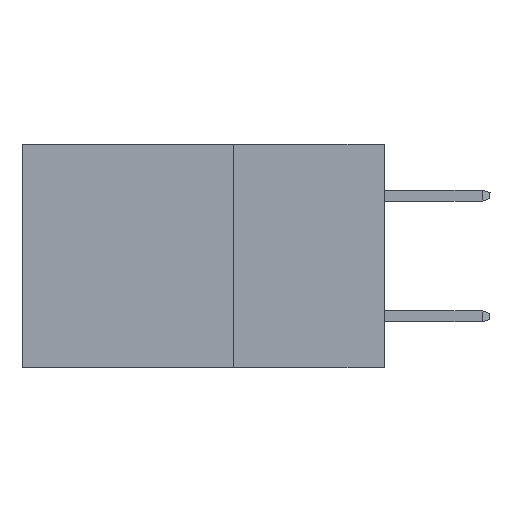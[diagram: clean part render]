
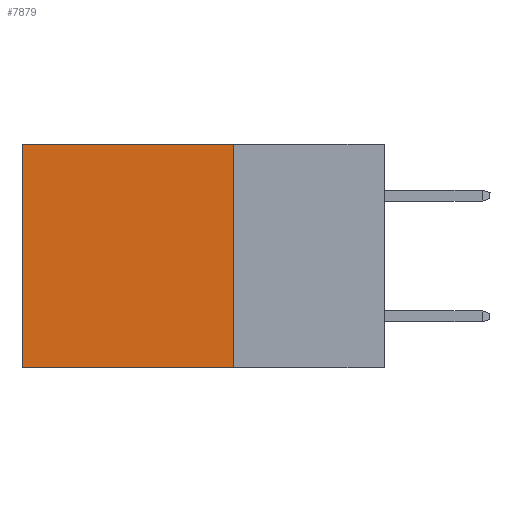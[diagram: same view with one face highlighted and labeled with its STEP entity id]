
A CAD part, left-side view. The second image highlights one B-rep face of the part: STEP entity #7879.
In plain terms, the highlighted planar face has unit normal (-1, 0, 0).
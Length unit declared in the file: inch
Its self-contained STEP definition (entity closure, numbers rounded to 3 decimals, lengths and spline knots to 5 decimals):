
#285 = VECTOR ( 'NONE', #1571, 39.37008 ) ;
#515 = VERTEX_POINT ( 'NONE', #2624 ) ;
#549 = CARTESIAN_POINT ( 'NONE',  ( 0.298, 0.6, -0.37 ) ) ;
#771 = FACE_OUTER_BOUND ( 'NONE', #9081, .T. ) ;
#797 = ORIENTED_EDGE ( 'NONE', *, *, #4668, .T. ) ;
#1075 = CARTESIAN_POINT ( 'NONE',  ( 0.298, 0.25, -0.37 ) ) ;
#1334 = CARTESIAN_POINT ( 'NONE',  ( 0.298, 0.25, 0. ) ) ;
#1498 = CARTESIAN_POINT ( 'NONE',  ( 0.298, 0.25, 0. ) ) ;
#1571 = DIRECTION ( 'NONE',  ( 0., 0., -1. ) ) ;
#1808 = EDGE_CURVE ( 'NONE', #4935, #515, #9360, .T. ) ;
#1875 = PLANE ( 'NONE',  #2362 ) ;
#2045 = DIRECTION ( 'NONE',  ( 0., 1., 0. ) ) ;
#2288 = LINE ( 'NONE', #7924, #6374 ) ;
#2362 = AXIS2_PLACEMENT_3D ( 'NONE', #1334, #10257, #8568 ) ;
#2490 = CARTESIAN_POINT ( 'NONE',  ( 0.298, 0.6, 0. ) ) ;
#2624 = CARTESIAN_POINT ( 'NONE',  ( 0.298, 0.25, -0.37 ) ) ;
#3165 = DIRECTION ( 'NONE',  ( 0., 1., 0. ) ) ;
#4533 = VECTOR ( 'NONE', #2045, 39.37008 ) ;
#4668 = EDGE_CURVE ( 'NONE', #4935, #5518, #2288, .T. ) ;
#4935 = VERTEX_POINT ( 'NONE', #9321 ) ;
#5134 = VERTEX_POINT ( 'NONE', #549 ) ;
#5518 = VERTEX_POINT ( 'NONE', #9917 ) ;
#5830 = ORIENTED_EDGE ( 'NONE', *, *, #1808, .F. ) ;
#6374 = VECTOR ( 'NONE', #3165, 39.37008 ) ;
#7879 = ADVANCED_FACE ( 'NONE', ( #771 ), #1875, .F. ) ;
#7924 = CARTESIAN_POINT ( 'NONE',  ( 0.298, 0.25, 0. ) ) ;
#8568 = DIRECTION ( 'NONE',  ( 0., 0., -1. ) ) ;
#8782 = ORIENTED_EDGE ( 'NONE', *, *, #9689, .T. ) ;
#9014 = DIRECTION ( 'NONE',  ( 0., 0., -1. ) ) ;
#9022 = LINE ( 'NONE', #2490, #9277 ) ;
#9081 = EDGE_LOOP ( 'NONE', ( #8782, #9554, #5830, #797 ) ) ;
#9277 = VECTOR ( 'NONE', #9014, 39.37008 ) ;
#9321 = CARTESIAN_POINT ( 'NONE',  ( 0.298, 0.25, 0. ) ) ;
#9360 = LINE ( 'NONE', #1498, #285 ) ;
#9554 = ORIENTED_EDGE ( 'NONE', *, *, #10515, .F. ) ;
#9689 = EDGE_CURVE ( 'NONE', #5518, #5134, #9022, .T. ) ;
#9917 = CARTESIAN_POINT ( 'NONE',  ( 0.298, 0.6, 0. ) ) ;
#10257 = DIRECTION ( 'NONE',  ( 1., 0., 0. ) ) ;
#10515 = EDGE_CURVE ( 'NONE', #515, #5134, #10545, .T. ) ;
#10545 = LINE ( 'NONE', #1075, #4533 ) ;
